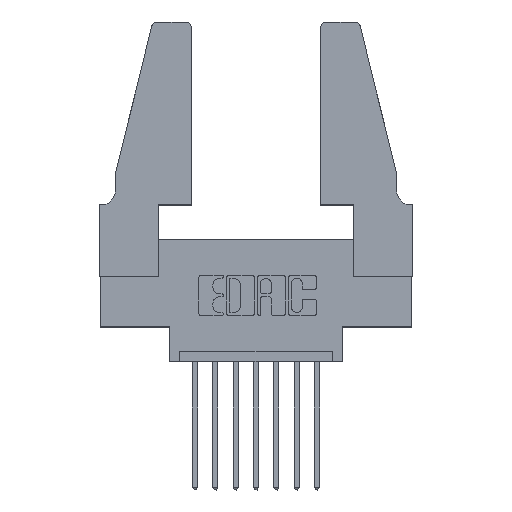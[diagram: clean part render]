
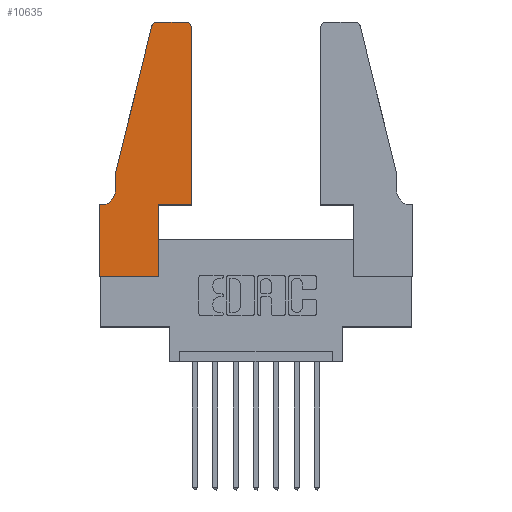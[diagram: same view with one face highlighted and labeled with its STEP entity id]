
A CAD part, top view. The second image highlights one B-rep face of the part: STEP entity #10635.
In plain terms, the highlighted planar face has unit normal (0, 0, 1).
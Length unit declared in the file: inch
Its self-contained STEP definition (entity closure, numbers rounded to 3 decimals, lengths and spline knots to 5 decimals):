
#11 = DIRECTION ( 'NONE',  ( 0., 1., 0. ) ) ;
#25 = VERTEX_POINT ( 'NONE', #6660 ) ;
#205 = VERTEX_POINT ( 'NONE', #9100 ) ;
#488 = ORIENTED_EDGE ( 'NONE', *, *, #5203, .T. ) ;
#725 = VECTOR ( 'NONE', #2849, 39.37008 ) ;
#886 = LINE ( 'NONE', #6585, #725 ) ;
#1079 = VECTOR ( 'NONE', #7391, 39.37008 ) ;
#1214 = CARTESIAN_POINT ( 'NONE',  ( 0.4205, 1.25, 0.37 ) ) ;
#1292 = CIRCLE ( 'NONE', #4325, 0.03 ) ;
#1629 = VECTOR ( 'NONE', #3765, 39.37008 ) ;
#1631 = CARTESIAN_POINT ( 'NONE',  ( 0.25487, 1.22718, 0.37 ) ) ;
#1639 = CARTESIAN_POINT ( 'NONE',  ( 0.2865, 0.35, 0.37 ) ) ;
#1666 = ORIENTED_EDGE ( 'NONE', *, *, #5606, .T. ) ;
#1704 = VERTEX_POINT ( 'NONE', #6577 ) ;
#1727 = LINE ( 'NONE', #9024, #8277 ) ;
#1764 = CARTESIAN_POINT ( 'NONE',  ( 0., 0., 0.37 ) ) ;
#1887 = ORIENTED_EDGE ( 'NONE', *, *, #6012, .T. ) ;
#1988 = ORIENTED_EDGE ( 'NONE', *, *, #11697, .T. ) ;
#2167 = CARTESIAN_POINT ( 'NONE',  ( 0.284, 1.22, 0.37 ) ) ;
#2203 = ORIENTED_EDGE ( 'NONE', *, *, #4313, .T. ) ;
#2220 = EDGE_CURVE ( 'NONE', #3649, #2359, #9531, .T. ) ;
#2226 = DIRECTION ( 'NONE',  ( 0., 0., 1. ) ) ;
#2303 = LINE ( 'NONE', #7570, #12063 ) ;
#2340 = VECTOR ( 'NONE', #8925, 39.37008 ) ;
#2359 = VERTEX_POINT ( 'NONE', #10314 ) ;
#2518 = CARTESIAN_POINT ( 'NONE',  ( 0.0055, 0.35, 0.37 ) ) ;
#2759 = ORIENTED_EDGE ( 'NONE', *, *, #3858, .T. ) ;
#2849 = DIRECTION ( 'NONE',  ( 1., 0., 0. ) ) ;
#2944 = CARTESIAN_POINT ( 'NONE',  ( 0.4505, 0.35, 0.37 ) ) ;
#3025 = VERTEX_POINT ( 'NONE', #9681 ) ;
#3132 = DIRECTION ( 'NONE',  ( 0., 0., 1. ) ) ;
#3335 = VERTEX_POINT ( 'NONE', #4627 ) ;
#3649 = VERTEX_POINT ( 'NONE', #1631 ) ;
#3765 = DIRECTION ( 'NONE',  ( 0., -1., 0. ) ) ;
#3858 = EDGE_CURVE ( 'NONE', #2359, #3335, #10515, .T. ) ;
#3877 = CARTESIAN_POINT ( 'NONE',  ( 0.2865, 0., 0.37 ) ) ;
#4000 = EDGE_CURVE ( 'NONE', #10245, #1704, #886, .T. ) ;
#4313 = EDGE_CURVE ( 'NONE', #9251, #10245, #7732, .T. ) ;
#4325 = AXIS2_PLACEMENT_3D ( 'NONE', #4793, #10278, #12306 ) ;
#4378 = CARTESIAN_POINT ( 'NONE',  ( 0.0755, 0.5, 0.37 ) ) ;
#4457 = CARTESIAN_POINT ( 'NONE',  ( 0.2865, 0.35, 0.37 ) ) ;
#4565 = DIRECTION ( 'NONE',  ( 1., 0., 0. ) ) ;
#4620 = DIRECTION ( 'NONE',  ( -1., 0., 0. ) ) ;
#4627 = CARTESIAN_POINT ( 'NONE',  ( 0.0755, 0.42, 0.37 ) ) ;
#4793 = CARTESIAN_POINT ( 'NONE',  ( 0.4205, 1.22, 0.37 ) ) ;
#4880 = DIRECTION ( 'NONE',  ( 1., 0., 0. ) ) ;
#4944 = EDGE_CURVE ( 'NONE', #3335, #10786, #12274, .T. ) ;
#5042 = VECTOR ( 'NONE', #11, 39.37008 ) ;
#5117 = AXIS2_PLACEMENT_3D ( 'NONE', #5451, #7422, #10182 ) ;
#5184 = EDGE_LOOP ( 'NONE', ( #8655, #1988, #10287, #2759, #11326, #1666, #8379, #6739, #2203, #9424, #488, #1887 ) ) ;
#5203 = EDGE_CURVE ( 'NONE', #1704, #205, #5779, .T. ) ;
#5310 = DIRECTION ( 'NONE',  ( -1., 0., 0. ) ) ;
#5451 = CARTESIAN_POINT ( 'NONE',  ( 0.0055, 0.42, 0.37 ) ) ;
#5606 = EDGE_CURVE ( 'NONE', #10786, #25, #1727, .T. ) ;
#5779 = LINE ( 'NONE', #2944, #5042 ) ;
#6012 = EDGE_CURVE ( 'NONE', #205, #8049, #1292, .T. ) ;
#6206 = LINE ( 'NONE', #7902, #2340 ) ;
#6577 = CARTESIAN_POINT ( 'NONE',  ( 0.4505, 0.35, 0.37 ) ) ;
#6585 = CARTESIAN_POINT ( 'NONE',  ( 0.4505, 0.35, 0.37 ) ) ;
#6660 = CARTESIAN_POINT ( 'NONE',  ( 0., 0.35, 0.37 ) ) ;
#6739 = ORIENTED_EDGE ( 'NONE', *, *, #12201, .T. ) ;
#6750 = CARTESIAN_POINT ( 'NONE',  ( 0.0755, 0.5, 0.37 ) ) ;
#7194 = VERTEX_POINT ( 'NONE', #1764 ) ;
#7391 = DIRECTION ( 'NONE',  ( -0.239, -0.971, 0. ) ) ;
#7422 = DIRECTION ( 'NONE',  ( 0., 0., -1. ) ) ;
#7570 = CARTESIAN_POINT ( 'NONE',  ( 0.2605, 1.25, 0.37 ) ) ;
#7732 = LINE ( 'NONE', #4457, #11246 ) ;
#7797 = EDGE_CURVE ( 'NONE', #8049, #3025, #2303, .T. ) ;
#7902 = CARTESIAN_POINT ( 'NONE',  ( 0., 0., 0.37 ) ) ;
#7922 = CARTESIAN_POINT ( 'NONE',  ( 0., 0.35, 0.37 ) ) ;
#7967 = AXIS2_PLACEMENT_3D ( 'NONE', #7922, #2226, #8905 ) ;
#8049 = VERTEX_POINT ( 'NONE', #1214 ) ;
#8069 = FACE_OUTER_BOUND ( 'NONE', #5184, .T. ) ;
#8127 = EDGE_CURVE ( 'NONE', #25, #7194, #6206, .T. ) ;
#8277 = VECTOR ( 'NONE', #5310, 39.37008 ) ;
#8379 = ORIENTED_EDGE ( 'NONE', *, *, #8127, .T. ) ;
#8655 = ORIENTED_EDGE ( 'NONE', *, *, #7797, .T. ) ;
#8905 = DIRECTION ( 'NONE',  ( 1., 0., 0. ) ) ;
#8925 = DIRECTION ( 'NONE',  ( 0., -1., 0. ) ) ;
#9024 = CARTESIAN_POINT ( 'NONE',  ( 0.0755, 0.35, 0.37 ) ) ;
#9100 = CARTESIAN_POINT ( 'NONE',  ( 0.4505, 1.22, 0.37 ) ) ;
#9251 = VERTEX_POINT ( 'NONE', #3877 ) ;
#9277 = CARTESIAN_POINT ( 'NONE',  ( 0., 0., 0.37 ) ) ;
#9424 = ORIENTED_EDGE ( 'NONE', *, *, #4000, .T. ) ;
#9484 = CIRCLE ( 'NONE', #9775, 0.03 ) ;
#9531 = LINE ( 'NONE', #4378, #1079 ) ;
#9681 = CARTESIAN_POINT ( 'NONE',  ( 0.284, 1.25, 0.37 ) ) ;
#9775 = AXIS2_PLACEMENT_3D ( 'NONE', #2167, #3132, #4880 ) ;
#9794 = LINE ( 'NONE', #9277, #10682 ) ;
#10182 = DIRECTION ( 'NONE',  ( -1., 0., 0. ) ) ;
#10219 = DIRECTION ( 'NONE',  ( 0., 1., 0. ) ) ;
#10245 = VERTEX_POINT ( 'NONE', #1639 ) ;
#10278 = DIRECTION ( 'NONE',  ( 0., 0., 1. ) ) ;
#10287 = ORIENTED_EDGE ( 'NONE', *, *, #2220, .T. ) ;
#10314 = CARTESIAN_POINT ( 'NONE',  ( 0.0755, 0.5, 0.37 ) ) ;
#10515 = LINE ( 'NONE', #6750, #1629 ) ;
#10635 = ADVANCED_FACE ( 'NONE', ( #8069 ), #11745, .T. ) ;
#10682 = VECTOR ( 'NONE', #4565, 39.37008 ) ;
#10786 = VERTEX_POINT ( 'NONE', #2518 ) ;
#11246 = VECTOR ( 'NONE', #10219, 39.37008 ) ;
#11326 = ORIENTED_EDGE ( 'NONE', *, *, #4944, .T. ) ;
#11697 = EDGE_CURVE ( 'NONE', #3025, #3649, #9484, .T. ) ;
#11745 = PLANE ( 'NONE',  #7967 ) ;
#12063 = VECTOR ( 'NONE', #4620, 39.37008 ) ;
#12201 = EDGE_CURVE ( 'NONE', #7194, #9251, #9794, .T. ) ;
#12274 = CIRCLE ( 'NONE', #5117, 0.07 ) ;
#12306 = DIRECTION ( 'NONE',  ( 1., 0., 0. ) ) ;
